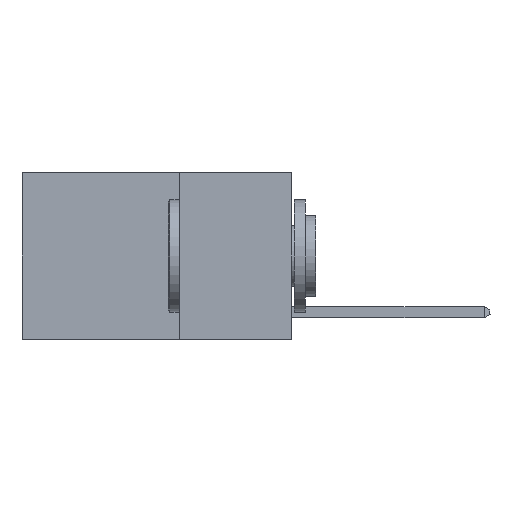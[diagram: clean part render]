
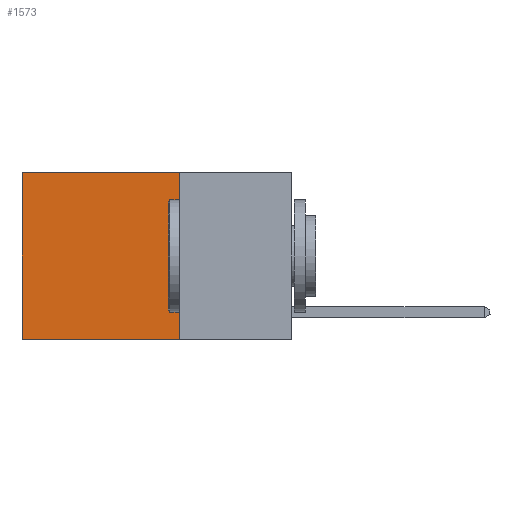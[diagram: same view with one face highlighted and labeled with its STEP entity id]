
A CAD part, left-side view. The second image highlights one B-rep face of the part: STEP entity #1573.
In plain terms, the highlighted planar face has unit normal (-1, 0, 0).
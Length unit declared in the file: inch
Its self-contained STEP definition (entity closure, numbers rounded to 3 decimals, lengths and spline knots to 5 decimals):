
#135 = LINE ( 'NONE', #7286, #13995 ) ;
#499 = EDGE_CURVE ( 'NONE', #5988, #6851, #10975, .T. ) ;
#818 = AXIS2_PLACEMENT_3D ( 'NONE', #7273, #8406, #9384 ) ;
#1037 = FACE_OUTER_BOUND ( 'NONE', #8461, .T. ) ;
#1573 = ADVANCED_FACE ( 'NONE', ( #1037 ), #5677, .F. ) ;
#1751 = CARTESIAN_POINT ( 'NONE',  ( 0.2625, 0.6, -0.37 ) ) ;
#2660 = VERTEX_POINT ( 'NONE', #1751 ) ;
#3538 = ORIENTED_EDGE ( 'NONE', *, *, #14163, .F. ) ;
#3775 = EDGE_CURVE ( 'NONE', #6851, #2660, #10056, .T. ) ;
#3937 = CARTESIAN_POINT ( 'NONE',  ( 0.2625, 0.25, 0. ) ) ;
#4395 = CARTESIAN_POINT ( 'NONE',  ( 0.2625, 0.25, -0.37 ) ) ;
#4719 = VERTEX_POINT ( 'NONE', #4395 ) ;
#4739 = CARTESIAN_POINT ( 'NONE',  ( 0.2625, 0.6, 0. ) ) ;
#5669 = ORIENTED_EDGE ( 'NONE', *, *, #3775, .T. ) ;
#5677 = PLANE ( 'NONE',  #818 ) ;
#5988 = VERTEX_POINT ( 'NONE', #11465 ) ;
#6634 = CARTESIAN_POINT ( 'NONE',  ( 0.2625, 0.25, -0.37 ) ) ;
#6743 = ORIENTED_EDGE ( 'NONE', *, *, #6826, .F. ) ;
#6826 = EDGE_CURVE ( 'NONE', #4719, #2660, #11033, .T. ) ;
#6851 = VERTEX_POINT ( 'NONE', #4739 ) ;
#7070 = ORIENTED_EDGE ( 'NONE', *, *, #499, .T. ) ;
#7273 = CARTESIAN_POINT ( 'NONE',  ( 0.2625, 0.25, 0. ) ) ;
#7286 = CARTESIAN_POINT ( 'NONE',  ( 0.2625, 0.25, 0. ) ) ;
#7564 = DIRECTION ( 'NONE',  ( 0., 1., 0. ) ) ;
#8406 = DIRECTION ( 'NONE',  ( 1., 0., 0. ) ) ;
#8461 = EDGE_LOOP ( 'NONE', ( #5669, #6743, #3538, #7070 ) ) ;
#8543 = VECTOR ( 'NONE', #11264, 39.37008 ) ;
#9384 = DIRECTION ( 'NONE',  ( 0., 0., -1. ) ) ;
#9904 = CARTESIAN_POINT ( 'NONE',  ( 0.2625, 0.6, 0. ) ) ;
#9976 = VECTOR ( 'NONE', #14534, 39.37008 ) ;
#10056 = LINE ( 'NONE', #9904, #9976 ) ;
#10975 = LINE ( 'NONE', #3937, #14928 ) ;
#11033 = LINE ( 'NONE', #6634, #8543 ) ;
#11264 = DIRECTION ( 'NONE',  ( 0., 1., 0. ) ) ;
#11465 = CARTESIAN_POINT ( 'NONE',  ( 0.2625, 0.25, 0. ) ) ;
#13113 = DIRECTION ( 'NONE',  ( 0., 0., -1. ) ) ;
#13995 = VECTOR ( 'NONE', #13113, 39.37008 ) ;
#14163 = EDGE_CURVE ( 'NONE', #5988, #4719, #135, .T. ) ;
#14534 = DIRECTION ( 'NONE',  ( 0., 0., -1. ) ) ;
#14928 = VECTOR ( 'NONE', #7564, 39.37008 ) ;
